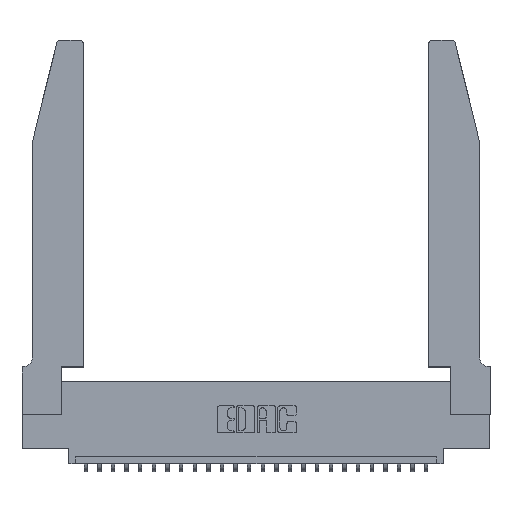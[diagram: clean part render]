
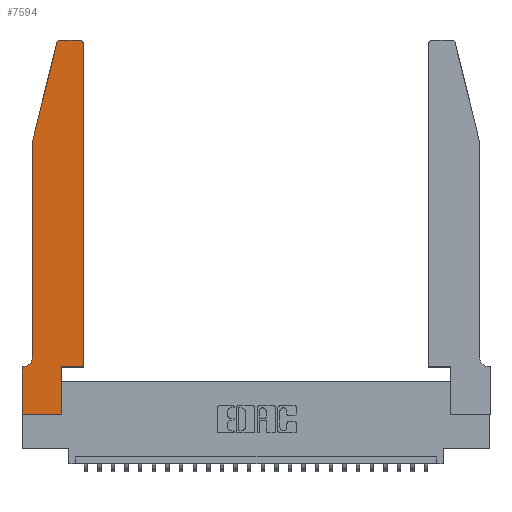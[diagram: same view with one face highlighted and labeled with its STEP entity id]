
A CAD part, top view. The second image highlights one B-rep face of the part: STEP entity #7594.
In plain terms, the highlighted planar face has unit normal (0, 0, 1).
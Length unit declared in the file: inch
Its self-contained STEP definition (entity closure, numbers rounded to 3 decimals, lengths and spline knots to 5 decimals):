
#243 = EDGE_CURVE ( 'NONE', #21822, #9685, #7311, .T. ) ;
#425 = VECTOR ( 'NONE', #20258, 39.37008 ) ;
#1046 = EDGE_CURVE ( 'NONE', #10361, #21822, #9197, .T. ) ;
#1554 = LINE ( 'NONE', #4687, #17329 ) ;
#1958 = CARTESIAN_POINT ( 'NONE',  ( 0., 0., 0.37 ) ) ;
#2088 = LINE ( 'NONE', #5823, #425 ) ;
#2157 = CARTESIAN_POINT ( 'NONE',  ( 0.0055, 0.35, 0.37 ) ) ;
#2425 = DIRECTION ( 'NONE',  ( 1., 0., 0. ) ) ;
#2516 = CARTESIAN_POINT ( 'NONE',  ( 0., 0.35, 0.37 ) ) ;
#2777 = CARTESIAN_POINT ( 'NONE',  ( 0.4505, 0.35, 0.37 ) ) ;
#3667 = DIRECTION ( 'NONE',  ( 0., 0., 1. ) ) ;
#3757 = CARTESIAN_POINT ( 'NONE',  ( 0.284, 2.72, 0.37 ) ) ;
#4216 = FACE_OUTER_BOUND ( 'NONE', #11904, .T. ) ;
#4587 = ORIENTED_EDGE ( 'NONE', *, *, #6248, .T. ) ;
#4687 = CARTESIAN_POINT ( 'NONE',  ( 0.4505, 0.35, 0.37 ) ) ;
#5068 = ORIENTED_EDGE ( 'NONE', *, *, #16982, .T. ) ;
#5543 = CIRCLE ( 'NONE', #22745, 0.07 ) ;
#5649 = ORIENTED_EDGE ( 'NONE', *, *, #24591, .T. ) ;
#5823 = CARTESIAN_POINT ( 'NONE',  ( 0.2605, 2.75, 0.37 ) ) ;
#5918 = LINE ( 'NONE', #2777, #16241 ) ;
#6057 = VECTOR ( 'NONE', #15705, 39.37008 ) ;
#6100 = DIRECTION ( 'NONE',  ( 0., -1., 0. ) ) ;
#6114 = LINE ( 'NONE', #14734, #16080 ) ;
#6246 = EDGE_CURVE ( 'NONE', #12074, #7652, #20779, .T. ) ;
#6248 = EDGE_CURVE ( 'NONE', #7652, #13343, #2088, .T. ) ;
#6433 = AXIS2_PLACEMENT_3D ( 'NONE', #22206, #9872, #16095 ) ;
#6505 = ORIENTED_EDGE ( 'NONE', *, *, #1046, .T. ) ;
#6517 = CARTESIAN_POINT ( 'NONE',  ( 0.284, 2.75, 0.37 ) ) ;
#6601 = CARTESIAN_POINT ( 'NONE',  ( 0., 0.35, 0.37 ) ) ;
#6952 = DIRECTION ( 'NONE',  ( 0., 0., 1. ) ) ;
#7218 = DIRECTION ( 'NONE',  ( 0., -1., 0. ) ) ;
#7305 = CARTESIAN_POINT ( 'NONE',  ( 0.0755, 2., 0.37 ) ) ;
#7311 = LINE ( 'NONE', #7305, #13109 ) ;
#7448 = ORIENTED_EDGE ( 'NONE', *, *, #243, .T. ) ;
#7594 = ADVANCED_FACE ( 'NONE', ( #4216 ), #8753, .T. ) ;
#7652 = VERTEX_POINT ( 'NONE', #16906 ) ;
#7710 = ORIENTED_EDGE ( 'NONE', *, *, #26612, .T. ) ;
#7879 = CARTESIAN_POINT ( 'NONE',  ( 0.0755, 0.35, 0.37 ) ) ;
#8753 = PLANE ( 'NONE',  #19070 ) ;
#8759 = VERTEX_POINT ( 'NONE', #23510 ) ;
#8787 = CARTESIAN_POINT ( 'NONE',  ( 0.0755, 2., 0.37 ) ) ;
#9006 = CARTESIAN_POINT ( 'NONE',  ( 0.0755, 2., 0.37 ) ) ;
#9029 = DIRECTION ( 'NONE',  ( 1., 0., 0. ) ) ;
#9197 = LINE ( 'NONE', #9006, #12106 ) ;
#9685 = VERTEX_POINT ( 'NONE', #15527 ) ;
#9872 = DIRECTION ( 'NONE',  ( 0., 0., 1. ) ) ;
#10012 = VECTOR ( 'NONE', #13106, 39.37008 ) ;
#10361 = VERTEX_POINT ( 'NONE', #17842 ) ;
#10730 = EDGE_CURVE ( 'NONE', #25795, #13946, #13414, .T. ) ;
#11462 = CARTESIAN_POINT ( 'NONE',  ( 0.0055, 0.42, 0.37 ) ) ;
#11756 = CARTESIAN_POINT ( 'NONE',  ( 0.2865, 0.35, 0.37 ) ) ;
#11904 = EDGE_LOOP ( 'NONE', ( #4587, #17866, #6505, #7448, #21624, #5068, #13777, #21930, #5649, #12124, #7710, #22900 ) ) ;
#12074 = VERTEX_POINT ( 'NONE', #23248 ) ;
#12106 = VECTOR ( 'NONE', #23318, 39.37008 ) ;
#12124 = ORIENTED_EDGE ( 'NONE', *, *, #13023, .T. ) ;
#12651 = AXIS2_PLACEMENT_3D ( 'NONE', #3757, #3667, #18073 ) ;
#12668 = VERTEX_POINT ( 'NONE', #23631 ) ;
#12889 = CIRCLE ( 'NONE', #12651, 0.03 ) ;
#13023 = EDGE_CURVE ( 'NONE', #26089, #8759, #5918, .T. ) ;
#13106 = DIRECTION ( 'NONE',  ( 0., 1., 0. ) ) ;
#13109 = VECTOR ( 'NONE', #7218, 39.37008 ) ;
#13343 = VERTEX_POINT ( 'NONE', #6517 ) ;
#13414 = LINE ( 'NONE', #1958, #23036 ) ;
#13532 = EDGE_CURVE ( 'NONE', #9685, #25690, #5543, .T. ) ;
#13777 = ORIENTED_EDGE ( 'NONE', *, *, #10730, .T. ) ;
#13946 = VERTEX_POINT ( 'NONE', #23497 ) ;
#14734 = CARTESIAN_POINT ( 'NONE',  ( 0., 0., 0.37 ) ) ;
#15192 = DIRECTION ( 'NONE',  ( 1., 0., 0. ) ) ;
#15527 = CARTESIAN_POINT ( 'NONE',  ( 0.0755, 0.42, 0.37 ) ) ;
#15705 = DIRECTION ( 'NONE',  ( -1., 0., 0. ) ) ;
#15737 = EDGE_CURVE ( 'NONE', #13343, #10361, #12889, .T. ) ;
#16080 = VECTOR ( 'NONE', #2425, 39.37008 ) ;
#16095 = DIRECTION ( 'NONE',  ( 1., 0., 0. ) ) ;
#16241 = VECTOR ( 'NONE', #15192, 39.37008 ) ;
#16906 = CARTESIAN_POINT ( 'NONE',  ( 0.4205, 2.75, 0.37 ) ) ;
#16982 = EDGE_CURVE ( 'NONE', #25690, #25795, #19259, .T. ) ;
#17329 = VECTOR ( 'NONE', #25023, 39.37008 ) ;
#17676 = DIRECTION ( 'NONE',  ( 0., 0., -1. ) ) ;
#17842 = CARTESIAN_POINT ( 'NONE',  ( 0.25487, 2.72718, 0.37 ) ) ;
#17866 = ORIENTED_EDGE ( 'NONE', *, *, #15737, .T. ) ;
#18073 = DIRECTION ( 'NONE',  ( 1., 0., 0. ) ) ;
#18724 = LINE ( 'NONE', #21202, #10012 ) ;
#19070 = AXIS2_PLACEMENT_3D ( 'NONE', #6601, #6952, #9029 ) ;
#19225 = EDGE_CURVE ( 'NONE', #13946, #12668, #6114, .T. ) ;
#19259 = LINE ( 'NONE', #7879, #6057 ) ;
#19764 = DIRECTION ( 'NONE',  ( -1., 0., 0. ) ) ;
#20258 = DIRECTION ( 'NONE',  ( -1., 0., 0. ) ) ;
#20779 = CIRCLE ( 'NONE', #6433, 0.03 ) ;
#21202 = CARTESIAN_POINT ( 'NONE',  ( 0.2865, 0.35, 0.37 ) ) ;
#21624 = ORIENTED_EDGE ( 'NONE', *, *, #13532, .T. ) ;
#21822 = VERTEX_POINT ( 'NONE', #8787 ) ;
#21930 = ORIENTED_EDGE ( 'NONE', *, *, #19225, .T. ) ;
#22206 = CARTESIAN_POINT ( 'NONE',  ( 0.4205, 2.72, 0.37 ) ) ;
#22745 = AXIS2_PLACEMENT_3D ( 'NONE', #11462, #17676, #19764 ) ;
#22900 = ORIENTED_EDGE ( 'NONE', *, *, #6246, .T. ) ;
#23036 = VECTOR ( 'NONE', #6100, 39.37008 ) ;
#23248 = CARTESIAN_POINT ( 'NONE',  ( 0.4505, 2.72, 0.37 ) ) ;
#23318 = DIRECTION ( 'NONE',  ( -0.239, -0.971, 0. ) ) ;
#23497 = CARTESIAN_POINT ( 'NONE',  ( 0., 0., 0.37 ) ) ;
#23510 = CARTESIAN_POINT ( 'NONE',  ( 0.4505, 0.35, 0.37 ) ) ;
#23631 = CARTESIAN_POINT ( 'NONE',  ( 0.2865, 0., 0.37 ) ) ;
#24591 = EDGE_CURVE ( 'NONE', #12668, #26089, #18724, .T. ) ;
#25023 = DIRECTION ( 'NONE',  ( 0., 1., 0. ) ) ;
#25690 = VERTEX_POINT ( 'NONE', #2157 ) ;
#25795 = VERTEX_POINT ( 'NONE', #2516 ) ;
#26089 = VERTEX_POINT ( 'NONE', #11756 ) ;
#26612 = EDGE_CURVE ( 'NONE', #8759, #12074, #1554, .T. ) ;
